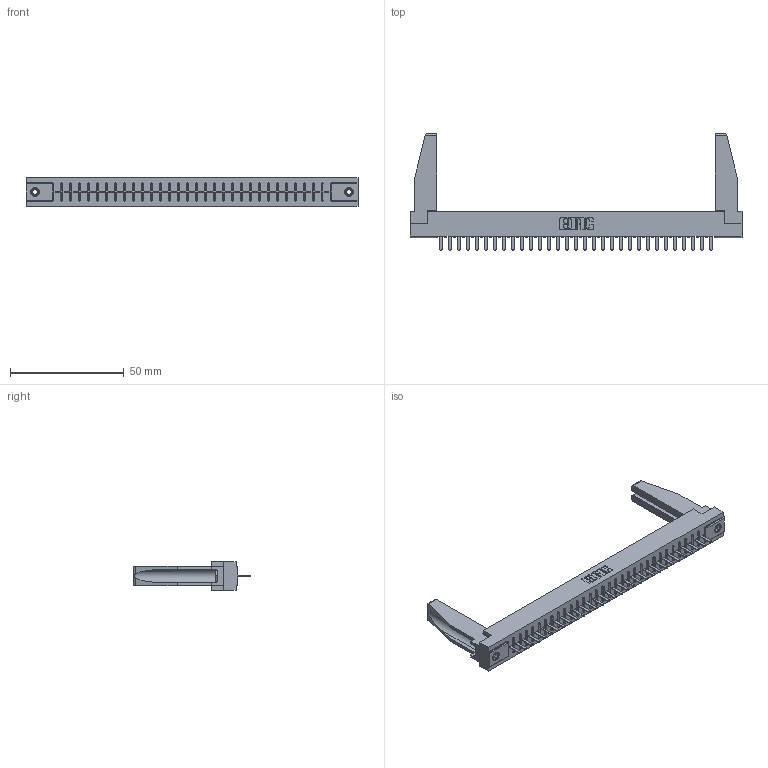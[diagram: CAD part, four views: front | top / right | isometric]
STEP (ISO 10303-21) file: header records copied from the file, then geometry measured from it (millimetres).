
FILE_DESCRIPTION (( 'STEP AP203' ), '1' );
FILE_NAME ('306-031-420-178.STEP', '2020-09-22T01:49:21', ( '' ), ( '' ), 'SwSTEP 2.0', 'SolidWorks 2020', '' );
FILE_SCHEMA (( 'CONFIG_CONTROL_DESIGN' ));
Length unit declared in the file: inch
Products named in the file (5): 306 Part_.156 Dia; 306-031-420-178; 307-220-078; 306-290-001_120; 345-250-001_345-250-001-102
Assembly tree (36 placements, depth 2):
  306-031-420-178
    306 Part_.156 Dia
    306-290-001_120  x31
    345-250-001_345-250-001-102  x2
    307-220-078  x2
Bounding box: 145.85 x 51.16 x 12.7 mm (x, y, z)
Volume: 20023.8 mm3; surface area: 20182.7 mm2
Topology: 36 solids, 36 shells, 2416 faces, 6753 edges, 4326 vertices
Faces by surface type: plane 1609, cylinder 667, sphere 124, cone 12, torus 4
Entity records: 32729 total; most frequent: CARTESIAN_POINT 5494, ORIENTED_EDGE 5404, DIRECTION 5370, EDGE_CURVE 2702, LINE 2110, VECTOR 2110, VERTEX_POINT 1712, AXIS2_PLACEMENT_3D 1630
